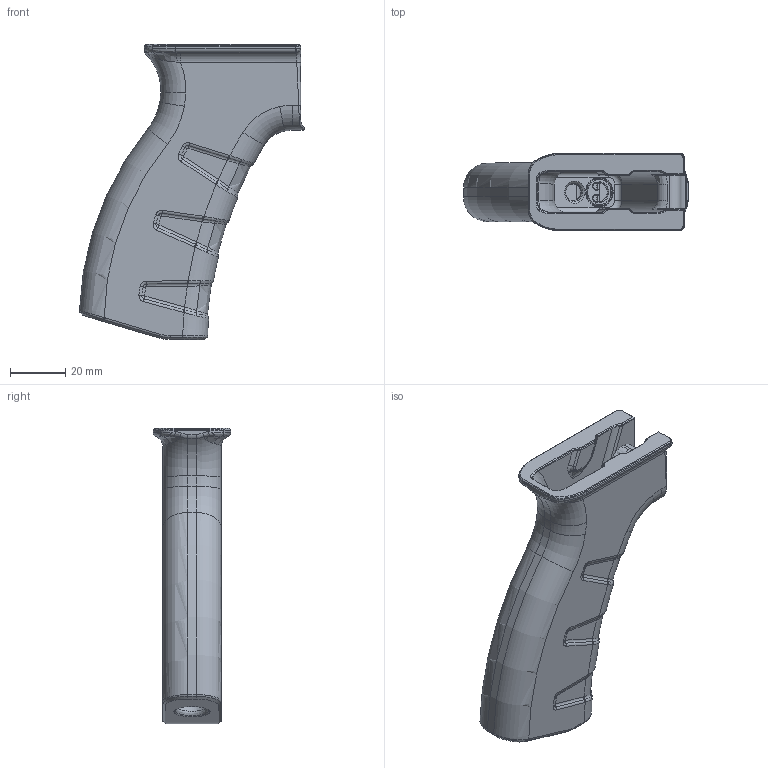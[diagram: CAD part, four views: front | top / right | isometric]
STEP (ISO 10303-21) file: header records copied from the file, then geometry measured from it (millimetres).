
FILE_DESCRIPTION(/* description */ (''),/* implementation_level */ '2;1');
FILE_NAME(/* name */ 'Wrapped Rib Grip.step',/* time_stamp */ '2021-09-20T01:27:35-04:00',/* author */ (''),/* organization */ (''),/* preprocessor_version */ 'ST-DEVELOPER v18.1',/* originating_system */ 'Autodesk Translation Framework v10.10.0.1391',/* authorisation */ '');
FILE_SCHEMA (('AUTOMOTIVE_DESIGN { 1 0 10303 214 3 1 1 }'));
Length unit declared in the file: millimetre
Products named in the file (1): Wrapped Rib Grip
Bounding box: 81.2 x 28 x 106.49 mm (x, y, z)
Volume: 51649.3 mm3; surface area: 25513.6 mm2
Topology: 1 solids, 1 shells, 659 faces, 1562 edges, 901 vertices
Faces by surface type: bspline 363, cylinder 140, torus 93, plane 58, cone 5
Full cylindrical faces by diameter (mm): 9 x1, 10.5 x1, 11 x1
Entity records: 26129 total; most frequent: CARTESIAN_POINT 12932, ORIENTED_EDGE 3100, DIRECTION 2168, EDGE_CURVE 1550, AXIS2_PLACEMENT_3D 928, VERTEX_POINT 901, EDGE_LOOP 669, FACE_OUTER_BOUND 659
